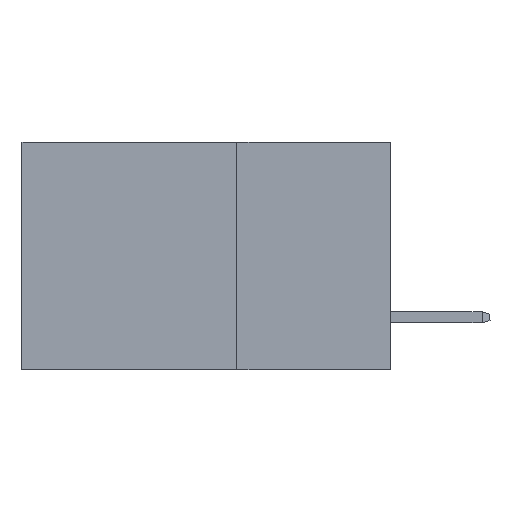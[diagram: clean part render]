
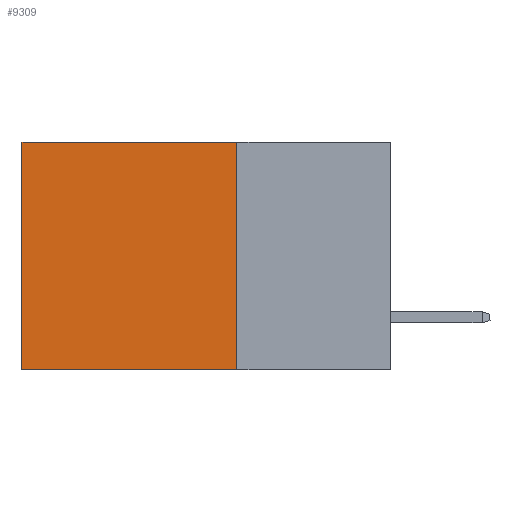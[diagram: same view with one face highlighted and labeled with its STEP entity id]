
A CAD part, left-side view. The second image highlights one B-rep face of the part: STEP entity #9309.
In plain terms, the highlighted planar face has unit normal (-1, 0, 0).
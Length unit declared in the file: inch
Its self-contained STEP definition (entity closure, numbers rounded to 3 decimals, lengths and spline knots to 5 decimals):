
#563 = ORIENTED_EDGE ( 'NONE', *, *, #1381, .F. ) ;
#1381 = EDGE_CURVE ( 'NONE', #22342, #9818, #10511, .T. ) ;
#1685 = VECTOR ( 'NONE', #3117, 39.37008 ) ;
#1907 = FACE_OUTER_BOUND ( 'NONE', #12042, .T. ) ;
#2019 = CARTESIAN_POINT ( 'NONE',  ( 0.2875, 0.25, 0. ) ) ;
#2317 = VECTOR ( 'NONE', #21507, 39.37008 ) ;
#2960 = CARTESIAN_POINT ( 'NONE',  ( 0.2875, 0.25, 0. ) ) ;
#3098 = EDGE_CURVE ( 'NONE', #9818, #16262, #6457, .T. ) ;
#3117 = DIRECTION ( 'NONE',  ( 0., 0., -1. ) ) ;
#3284 = VECTOR ( 'NONE', #18569, 39.37008 ) ;
#3649 = DIRECTION ( 'NONE',  ( 1., 0., 0. ) ) ;
#4964 = CARTESIAN_POINT ( 'NONE',  ( 0.2875, 0.25, -0.37 ) ) ;
#5352 = ORIENTED_EDGE ( 'NONE', *, *, #3098, .F. ) ;
#6457 = LINE ( 'NONE', #9606, #2317 ) ;
#8007 = LINE ( 'NONE', #2960, #3284 ) ;
#8933 = PLANE ( 'NONE',  #13444 ) ;
#9042 = EDGE_CURVE ( 'NONE', #22342, #15053, #8007, .T. ) ;
#9309 = ADVANCED_FACE ( 'NONE', ( #1907 ), #8933, .F. ) ;
#9548 = LINE ( 'NONE', #10065, #18112 ) ;
#9606 = CARTESIAN_POINT ( 'NONE',  ( 0.2875, 0.25, -0.37 ) ) ;
#9818 = VERTEX_POINT ( 'NONE', #4964 ) ;
#10065 = CARTESIAN_POINT ( 'NONE',  ( 0.2875, 0.6, 0. ) ) ;
#10511 = LINE ( 'NONE', #13627, #1685 ) ;
#12042 = EDGE_LOOP ( 'NONE', ( #21257, #5352, #563, #15545 ) ) ;
#13444 = AXIS2_PLACEMENT_3D ( 'NONE', #14131, #3649, #15851 ) ;
#13627 = CARTESIAN_POINT ( 'NONE',  ( 0.2875, 0.25, 0. ) ) ;
#14131 = CARTESIAN_POINT ( 'NONE',  ( 0.2875, 0.25, 0. ) ) ;
#15053 = VERTEX_POINT ( 'NONE', #22161 ) ;
#15545 = ORIENTED_EDGE ( 'NONE', *, *, #9042, .T. ) ;
#15851 = DIRECTION ( 'NONE',  ( 0., 0., -1. ) ) ;
#16262 = VERTEX_POINT ( 'NONE', #17281 ) ;
#17281 = CARTESIAN_POINT ( 'NONE',  ( 0.2875, 0.6, -0.37 ) ) ;
#18112 = VECTOR ( 'NONE', #18557, 39.37008 ) ;
#18557 = DIRECTION ( 'NONE',  ( 0., 0., -1. ) ) ;
#18569 = DIRECTION ( 'NONE',  ( 0., 1., 0. ) ) ;
#19077 = EDGE_CURVE ( 'NONE', #15053, #16262, #9548, .T. ) ;
#21257 = ORIENTED_EDGE ( 'NONE', *, *, #19077, .T. ) ;
#21507 = DIRECTION ( 'NONE',  ( 0., 1., 0. ) ) ;
#22161 = CARTESIAN_POINT ( 'NONE',  ( 0.2875, 0.6, 0. ) ) ;
#22342 = VERTEX_POINT ( 'NONE', #2019 ) ;
